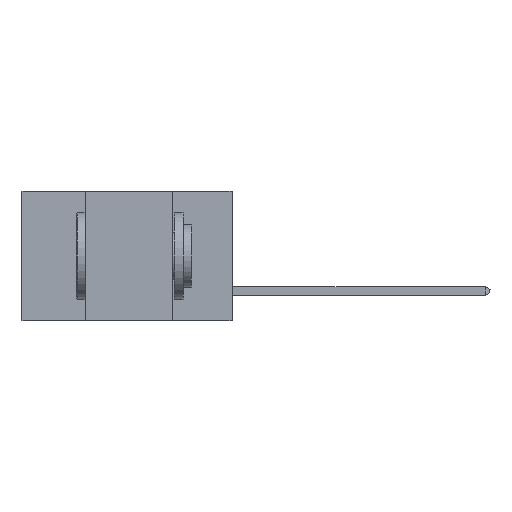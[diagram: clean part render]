
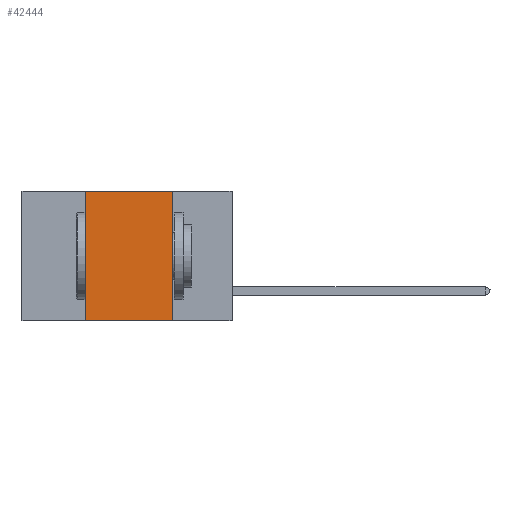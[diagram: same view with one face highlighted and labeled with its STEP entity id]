
A CAD part, left-side view. The second image highlights one B-rep face of the part: STEP entity #42444.
In plain terms, the highlighted planar face has unit normal (-1, 0, 0).
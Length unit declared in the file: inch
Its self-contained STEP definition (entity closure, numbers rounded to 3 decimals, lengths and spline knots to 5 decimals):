
#793 = DIRECTION ( 'NONE',  ( 0., 0., 1. ) ) ;
#1853 = CARTESIAN_POINT ( 'NONE',  ( 0., 0.42, -0.37 ) ) ;
#5306 = ORIENTED_EDGE ( 'NONE', *, *, #35189, .T. ) ;
#5368 = DIRECTION ( 'NONE',  ( 0., 0., -1. ) ) ;
#6487 = ORIENTED_EDGE ( 'NONE', *, *, #22306, .F. ) ;
#6604 = LINE ( 'NONE', #27223, #9707 ) ;
#6949 = VECTOR ( 'NONE', #37959, 39.37008 ) ;
#9707 = VECTOR ( 'NONE', #30979, 39.37008 ) ;
#13328 = EDGE_LOOP ( 'NONE', ( #6487, #13655, #37960, #5306 ) ) ;
#13655 = ORIENTED_EDGE ( 'NONE', *, *, #22985, .F. ) ;
#15225 = VERTEX_POINT ( 'NONE', #1853 ) ;
#15632 = VECTOR ( 'NONE', #793, 39.37008 ) ;
#15853 = LINE ( 'NONE', #24234, #6949 ) ;
#17780 = CARTESIAN_POINT ( 'NONE',  ( 0., 0.42, 0. ) ) ;
#22306 = EDGE_CURVE ( 'NONE', #30969, #35886, #6604, .T. ) ;
#22985 = EDGE_CURVE ( 'NONE', #29741, #30969, #37927, .T. ) ;
#24234 = CARTESIAN_POINT ( 'NONE',  ( 0., 0.6, -0.37 ) ) ;
#24529 = LINE ( 'NONE', #17780, #15632 ) ;
#26236 = EDGE_CURVE ( 'NONE', #15225, #29741, #24529, .T. ) ;
#27223 = CARTESIAN_POINT ( 'NONE',  ( 0., 0.17, 0. ) ) ;
#29201 = PLANE ( 'NONE',  #39394 ) ;
#29741 = VERTEX_POINT ( 'NONE', #37894 ) ;
#30969 = VERTEX_POINT ( 'NONE', #40234 ) ;
#30979 = DIRECTION ( 'NONE',  ( 0., 0., -1. ) ) ;
#33519 = CARTESIAN_POINT ( 'NONE',  ( 0., 0.6, 0. ) ) ;
#34142 = FACE_OUTER_BOUND ( 'NONE', #13328, .T. ) ;
#34785 = VECTOR ( 'NONE', #36908, 39.37008 ) ;
#35189 = EDGE_CURVE ( 'NONE', #15225, #35886, #15853, .T. ) ;
#35886 = VERTEX_POINT ( 'NONE', #40975 ) ;
#35940 = CARTESIAN_POINT ( 'NONE',  ( 0., 0.6, 0. ) ) ;
#36908 = DIRECTION ( 'NONE',  ( 0., -1., 0. ) ) ;
#37894 = CARTESIAN_POINT ( 'NONE',  ( 0., 0.42, 0. ) ) ;
#37927 = LINE ( 'NONE', #33519, #34785 ) ;
#37959 = DIRECTION ( 'NONE',  ( 0., -1., 0. ) ) ;
#37960 = ORIENTED_EDGE ( 'NONE', *, *, #26236, .F. ) ;
#39394 = AXIS2_PLACEMENT_3D ( 'NONE', #35940, #42088, #5368 ) ;
#40234 = CARTESIAN_POINT ( 'NONE',  ( 0., 0.17, 0. ) ) ;
#40975 = CARTESIAN_POINT ( 'NONE',  ( 0., 0.17, -0.37 ) ) ;
#42088 = DIRECTION ( 'NONE',  ( 1., 0., 0. ) ) ;
#42444 = ADVANCED_FACE ( 'NONE', ( #34142 ), #29201, .F. ) ;
